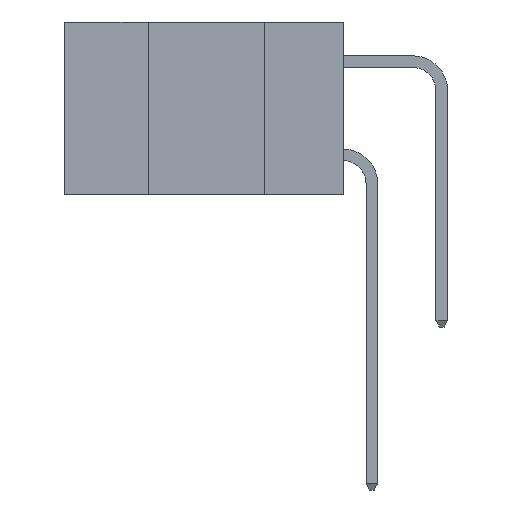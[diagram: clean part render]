
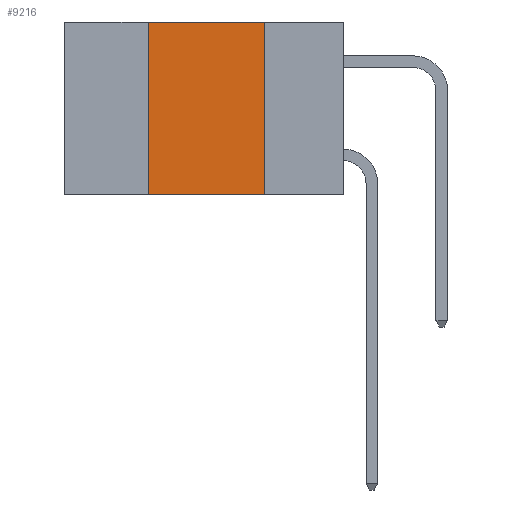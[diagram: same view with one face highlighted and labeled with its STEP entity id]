
A CAD part, left-side view. The second image highlights one B-rep face of the part: STEP entity #9216.
In plain terms, the highlighted planar face has unit normal (-1, 0, 0).
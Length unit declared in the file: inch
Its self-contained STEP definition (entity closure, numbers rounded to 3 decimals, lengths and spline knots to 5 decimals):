
#74 = CARTESIAN_POINT ( 'NONE',  ( 0., 0.17, 0. ) ) ;
#685 = LINE ( 'NONE', #9662, #7907 ) ;
#834 = PLANE ( 'NONE',  #10115 ) ;
#1170 = VECTOR ( 'NONE', #5613, 39.37008 ) ;
#1297 = EDGE_CURVE ( 'NONE', #8089, #1708, #685, .T. ) ;
#1708 = VERTEX_POINT ( 'NONE', #74 ) ;
#2583 = ORIENTED_EDGE ( 'NONE', *, *, #1297, .F. ) ;
#3294 = CARTESIAN_POINT ( 'NONE',  ( 0., 0.6, -0.37 ) ) ;
#4406 = LINE ( 'NONE', #6441, #12050 ) ;
#4771 = DIRECTION ( 'NONE',  ( 0., -1., 0. ) ) ;
#5177 = EDGE_CURVE ( 'NONE', #1708, #10051, #4406, .T. ) ;
#5511 = CARTESIAN_POINT ( 'NONE',  ( 0., 0.42, 0. ) ) ;
#5613 = DIRECTION ( 'NONE',  ( 0., 0., 1. ) ) ;
#5869 = EDGE_LOOP ( 'NONE', ( #12418, #2583, #5877, #7717 ) ) ;
#5877 = ORIENTED_EDGE ( 'NONE', *, *, #17770, .F. ) ;
#6165 = LINE ( 'NONE', #3294, #12858 ) ;
#6441 = CARTESIAN_POINT ( 'NONE',  ( 0., 0.17, -0.37 ) ) ;
#6621 = DIRECTION ( 'NONE',  ( 1., 0., 0. ) ) ;
#7406 = DIRECTION ( 'NONE',  ( 0., 0., -1. ) ) ;
#7717 = ORIENTED_EDGE ( 'NONE', *, *, #10349, .T. ) ;
#7907 = VECTOR ( 'NONE', #9195, 39.37008 ) ;
#8089 = VERTEX_POINT ( 'NONE', #5511 ) ;
#8818 = LINE ( 'NONE', #15528, #1170 ) ;
#9195 = DIRECTION ( 'NONE',  ( 0., -1., 0. ) ) ;
#9216 = ADVANCED_FACE ( 'NONE', ( #17634 ), #834, .F. ) ;
#9662 = CARTESIAN_POINT ( 'NONE',  ( 0., 0.6, 0. ) ) ;
#10051 = VERTEX_POINT ( 'NONE', #18198 ) ;
#10115 = AXIS2_PLACEMENT_3D ( 'NONE', #15123, #6621, #16485 ) ;
#10349 = EDGE_CURVE ( 'NONE', #11150, #10051, #6165, .T. ) ;
#11150 = VERTEX_POINT ( 'NONE', #12325 ) ;
#12050 = VECTOR ( 'NONE', #7406, 39.37008 ) ;
#12325 = CARTESIAN_POINT ( 'NONE',  ( 0., 0.42, -0.37 ) ) ;
#12418 = ORIENTED_EDGE ( 'NONE', *, *, #5177, .F. ) ;
#12858 = VECTOR ( 'NONE', #4771, 39.37008 ) ;
#15123 = CARTESIAN_POINT ( 'NONE',  ( 0., 0.6, 0. ) ) ;
#15528 = CARTESIAN_POINT ( 'NONE',  ( 0., 0.42, -0.37 ) ) ;
#16485 = DIRECTION ( 'NONE',  ( 0., 0., -1. ) ) ;
#17634 = FACE_OUTER_BOUND ( 'NONE', #5869, .T. ) ;
#17770 = EDGE_CURVE ( 'NONE', #11150, #8089, #8818, .T. ) ;
#18198 = CARTESIAN_POINT ( 'NONE',  ( 0., 0.17, -0.37 ) ) ;
